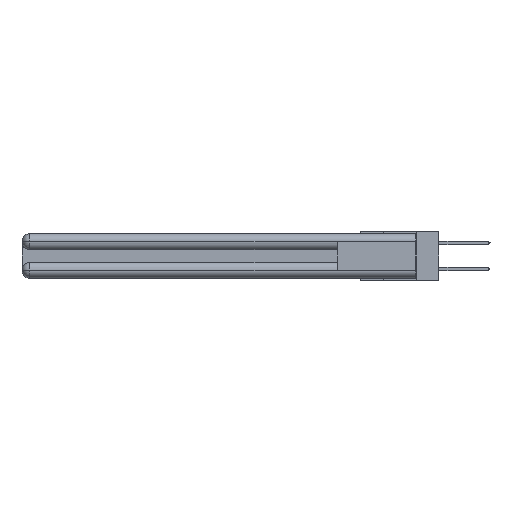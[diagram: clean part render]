
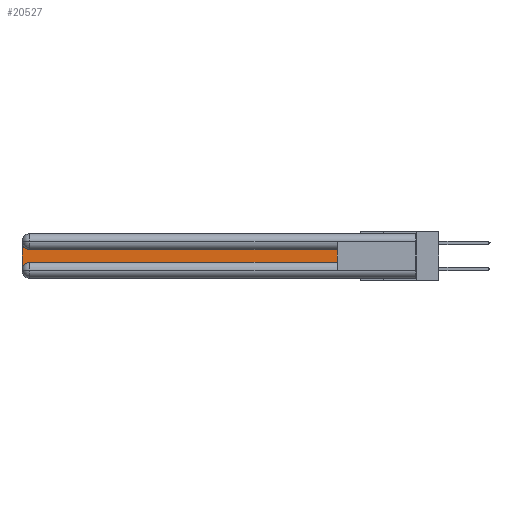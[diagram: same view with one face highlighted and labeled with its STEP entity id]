
A CAD part, left-side view. The second image highlights one B-rep face of the part: STEP entity #20527.
In plain terms, the highlighted planar face has unit normal (-1, 0, 0).
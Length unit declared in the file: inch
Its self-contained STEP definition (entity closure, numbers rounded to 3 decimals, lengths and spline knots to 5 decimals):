
#320 = CARTESIAN_POINT ( 'NONE',  ( 0.075, 0.6, -0.2175 ) ) ;
#1023 = DIRECTION ( 'NONE',  ( 1., 0., 0. ) ) ;
#1496 = DIRECTION ( 'NONE',  ( 0., -1., 0. ) ) ;
#1640 = CARTESIAN_POINT ( 'NONE',  ( 0.075, 2.94, -0.2775 ) ) ;
#2710 = CARTESIAN_POINT ( 'NONE',  ( 0.075, 2.94, -0.2175 ) ) ;
#2784 = ORIENTED_EDGE ( 'NONE', *, *, #20481, .T. ) ;
#3888 = AXIS2_PLACEMENT_3D ( 'NONE', #27252, #1023, #17860 ) ;
#3896 = CARTESIAN_POINT ( 'NONE',  ( 0.075, 0.6, -0.1225 ) ) ;
#4071 = DIRECTION ( 'NONE',  ( 0., 0., -1. ) ) ;
#4751 = CARTESIAN_POINT ( 'NONE',  ( 0.075, 2.94, -0.1225 ) ) ;
#5920 = VERTEX_POINT ( 'NONE', #4751 ) ;
#5953 = VERTEX_POINT ( 'NONE', #320 ) ;
#6181 = VECTOR ( 'NONE', #1496, 39.37008 ) ;
#7460 = VERTEX_POINT ( 'NONE', #3896 ) ;
#7667 = CARTESIAN_POINT ( 'NONE',  ( 0.075, 0.6, -0.1225 ) ) ;
#7709 = DIRECTION ( 'NONE',  ( 0., 0., -1. ) ) ;
#7878 = DIRECTION ( 'NONE',  ( 0., 1., 0. ) ) ;
#8592 = PLANE ( 'NONE',  #3888 ) ;
#8790 = CARTESIAN_POINT ( 'NONE',  ( 0.075, 3., -0.2775 ) ) ;
#10827 = DIRECTION ( 'NONE',  ( 1., 0., 0. ) ) ;
#10829 = DIRECTION ( 'NONE',  ( 0., 0., -1. ) ) ;
#10934 = EDGE_CURVE ( 'NONE', #5953, #7460, #30396, .T. ) ;
#11063 = VERTEX_POINT ( 'NONE', #2710 ) ;
#11876 = CIRCLE ( 'NONE', #26489, 0.06 ) ;
#12118 = LINE ( 'NONE', #7667, #30376 ) ;
#13256 = VECTOR ( 'NONE', #10829, 39.37008 ) ;
#13557 = CARTESIAN_POINT ( 'NONE',  ( 0.075, 0.6, -0.2175 ) ) ;
#14635 = EDGE_LOOP ( 'NONE', ( #2784, #21594, #19278, #22683, #15758, #20873 ) ) ;
#14743 = VECTOR ( 'NONE', #20091, 39.37008 ) ;
#15758 = ORIENTED_EDGE ( 'NONE', *, *, #26193, .T. ) ;
#16589 = EDGE_CURVE ( 'NONE', #21460, #26146, #17754, .T. ) ;
#17694 = CARTESIAN_POINT ( 'NONE',  ( 0.075, 3., -0.2175 ) ) ;
#17708 = CARTESIAN_POINT ( 'NONE',  ( 0.075, 0.6, -0.2175 ) ) ;
#17754 = LINE ( 'NONE', #17694, #13256 ) ;
#17860 = DIRECTION ( 'NONE',  ( 0., 0., -1. ) ) ;
#19278 = ORIENTED_EDGE ( 'NONE', *, *, #16589, .T. ) ;
#20091 = DIRECTION ( 'NONE',  ( 0., 0., 1. ) ) ;
#20481 = EDGE_CURVE ( 'NONE', #7460, #5920, #12118, .T. ) ;
#20527 = ADVANCED_FACE ( 'NONE', ( #21061 ), #8592, .F. ) ;
#20873 = ORIENTED_EDGE ( 'NONE', *, *, #10934, .T. ) ;
#21061 = FACE_OUTER_BOUND ( 'NONE', #14635, .T. ) ;
#21460 = VERTEX_POINT ( 'NONE', #22769 ) ;
#21594 = ORIENTED_EDGE ( 'NONE', *, *, #30641, .T. ) ;
#21988 = CARTESIAN_POINT ( 'NONE',  ( 0.075, 2.94, -0.0625 ) ) ;
#22683 = ORIENTED_EDGE ( 'NONE', *, *, #25117, .T. ) ;
#22769 = CARTESIAN_POINT ( 'NONE',  ( 0.075, 3., -0.0625 ) ) ;
#24395 = DIRECTION ( 'NONE',  ( 1., 0., 0. ) ) ;
#25117 = EDGE_CURVE ( 'NONE', #26146, #11063, #11876, .T. ) ;
#25917 = LINE ( 'NONE', #13557, #6181 ) ;
#26146 = VERTEX_POINT ( 'NONE', #8790 ) ;
#26193 = EDGE_CURVE ( 'NONE', #11063, #5953, #25917, .T. ) ;
#26489 = AXIS2_PLACEMENT_3D ( 'NONE', #1640, #10827, #4071 ) ;
#26837 = CIRCLE ( 'NONE', #29017, 0.06 ) ;
#27252 = CARTESIAN_POINT ( 'NONE',  ( 0.075, 3., -0.1225 ) ) ;
#29017 = AXIS2_PLACEMENT_3D ( 'NONE', #21988, #24395, #7709 ) ;
#30376 = VECTOR ( 'NONE', #7878, 39.37008 ) ;
#30396 = LINE ( 'NONE', #17708, #14743 ) ;
#30641 = EDGE_CURVE ( 'NONE', #5920, #21460, #26837, .T. ) ;
